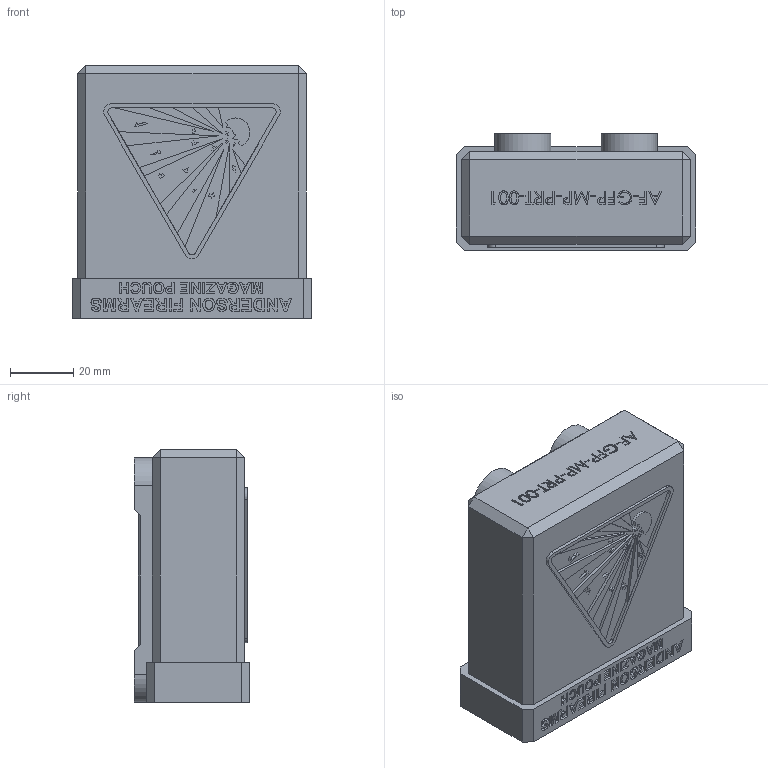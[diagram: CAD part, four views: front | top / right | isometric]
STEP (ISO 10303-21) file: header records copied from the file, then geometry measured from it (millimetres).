
FILE_DESCRIPTION (( 'STEP AP203' ), '1' );
FILE_NAME ('AF-GFP-MP-PRT-001-STEP.STEP', '2020-07-31T12:51:08', ( '' ), ( '' ), 'SwSTEP 2.0', 'SolidWorks 2018', '' );
FILE_SCHEMA (( 'CONFIG_CONTROL_DESIGN' ));
Length unit declared in the file: inch
Products named in the file (1): AF-GFP-MP-PRT-001-STEP
Bounding box: 75.98 x 36.72 x 80.01 mm (x, y, z)
Volume: 59398.4 mm3; surface area: 40344 mm2
Topology: 1 solids, 1 shells, 1076 faces, 2929 edges, 1940 vertices
Faces by surface type: plane 812, bspline 174, cylinder 82, cone 8
Entity records: 45930 total; most frequent: CARTESIAN_POINT 20092, ORIENTED_EDGE 5858, DIRECTION 4377, EDGE_CURVE 2929, LINE 2367, VECTOR 2367, VERTEX_POINT 1940, EDGE_LOOP 1161
